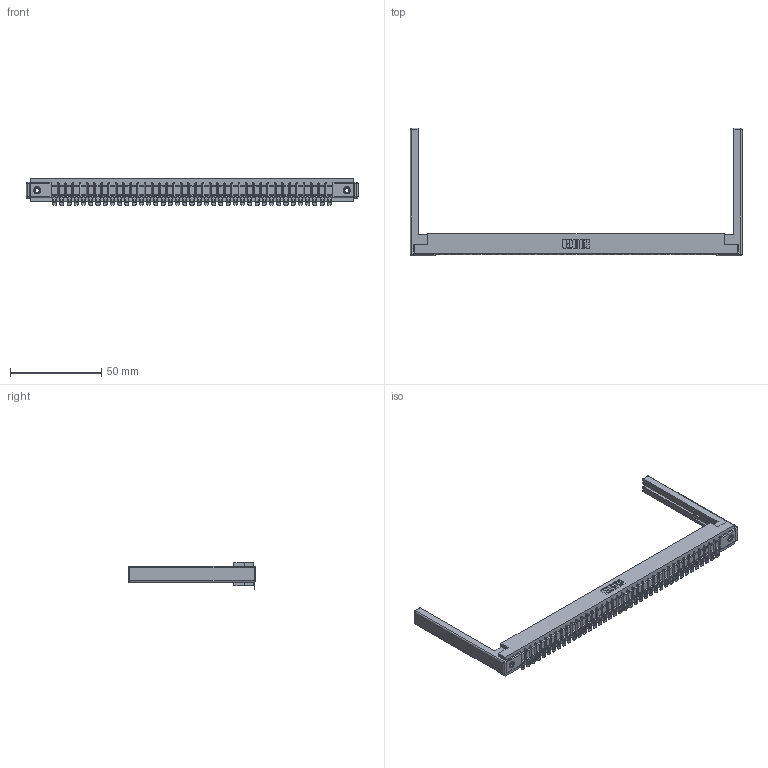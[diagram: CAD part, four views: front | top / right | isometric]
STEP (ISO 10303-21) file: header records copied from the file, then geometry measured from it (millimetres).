
FILE_DESCRIPTION (( 'STEP AP203' ), '1' );
FILE_NAME ('357-039-554-168.STEP', '2019-09-17T08:40:37', ( '' ), ( '' ), 'SwSTEP 2.0', 'SolidWorks 2016', '' );
FILE_SCHEMA (( 'CONFIG_CONTROL_DESIGN' ));
Length unit declared in the file: inch
Products named in the file (5): 357-039-554-168; 307-220-068; 345-250-001_345-250-001-102; 307-290-002_554; 307 Part_.156 Dia Mounting Holes
Assembly tree (44 placements, depth 2):
  357-039-554-168
    307 Part_.156 Dia Mounting Holes
    307-290-002_554  x39
    307-220-068  x2
    345-250-001_345-250-001-102  x2
Bounding box: 181.97 x 69.98 x 14.52 mm (x, y, z)
Volume: 23841.9 mm3; surface area: 28519.2 mm2
Topology: 44 solids, 44 shells, 3471 faces, 10580 edges, 6924 vertices
Faces by surface type: plane 1952, cylinder 1415, sphere 88, cone 12, torus 4
Entity records: 37528 total; most frequent: CARTESIAN_POINT 6295, ORIENTED_EDGE 6274, DIRECTION 6141, EDGE_CURVE 3137, LINE 2393, VECTOR 2393, VERTEX_POINT 2028, AXIS2_PLACEMENT_3D 1874
